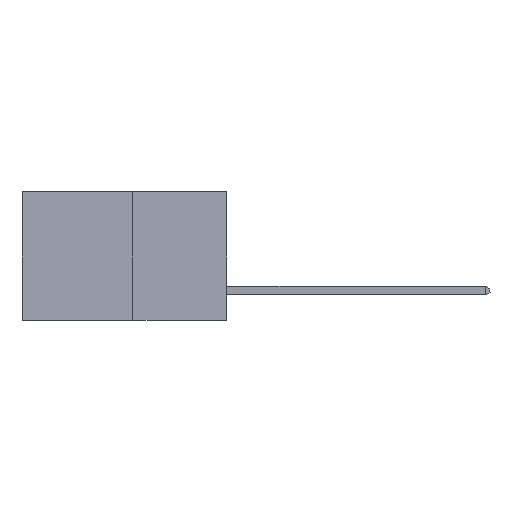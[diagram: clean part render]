
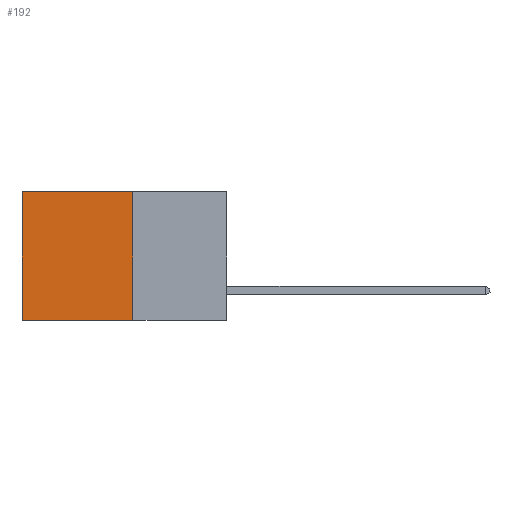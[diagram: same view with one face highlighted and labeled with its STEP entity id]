
A CAD part, left-side view. The second image highlights one B-rep face of the part: STEP entity #192.
In plain terms, the highlighted planar face has unit normal (-1, 0, 0).
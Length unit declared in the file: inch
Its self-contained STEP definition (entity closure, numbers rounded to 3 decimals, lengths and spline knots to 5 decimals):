
#144 = DIRECTION ( 'NONE',  ( 0., 0., -1. ) ) ;
#192 = ADVANCED_FACE ( 'NONE', ( #1609 ), #7700, .F. ) ;
#732 = EDGE_CURVE ( 'NONE', #3911, #3355, #3521, .T. ) ;
#922 = CARTESIAN_POINT ( 'NONE',  ( 0.277, 0.27, -0.37 ) ) ;
#1063 = CARTESIAN_POINT ( 'NONE',  ( 0.277, 0.59, -0.37 ) ) ;
#1507 = VERTEX_POINT ( 'NONE', #5740 ) ;
#1609 = FACE_OUTER_BOUND ( 'NONE', #6338, .T. ) ;
#2137 = LINE ( 'NONE', #7015, #6208 ) ;
#2222 = VECTOR ( 'NONE', #8670, 39.37008 ) ;
#3355 = VERTEX_POINT ( 'NONE', #5655 ) ;
#3521 = LINE ( 'NONE', #922, #7476 ) ;
#3780 = LINE ( 'NONE', #1063, #7697 ) ;
#3911 = VERTEX_POINT ( 'NONE', #6805 ) ;
#4600 = CARTESIAN_POINT ( 'NONE',  ( 0.277, 0.27, -0.37 ) ) ;
#5013 = ORIENTED_EDGE ( 'NONE', *, *, #8969, .T. ) ;
#5041 = CARTESIAN_POINT ( 'NONE',  ( 0.277, 0.27, 0. ) ) ;
#5655 = CARTESIAN_POINT ( 'NONE',  ( 0.277, 0.59, -0.37 ) ) ;
#5740 = CARTESIAN_POINT ( 'NONE',  ( 0.277, 0.27, 0. ) ) ;
#5811 = DIRECTION ( 'NONE',  ( 0., 0., -1. ) ) ;
#6208 = VECTOR ( 'NONE', #7864, 39.37008 ) ;
#6263 = AXIS2_PLACEMENT_3D ( 'NONE', #4600, #8094, #5811 ) ;
#6338 = EDGE_LOOP ( 'NONE', ( #5013, #8793, #6616, #9136 ) ) ;
#6616 = ORIENTED_EDGE ( 'NONE', *, *, #7579, .F. ) ;
#6711 = VERTEX_POINT ( 'NONE', #7146 ) ;
#6805 = CARTESIAN_POINT ( 'NONE',  ( 0.277, 0.27, -0.37 ) ) ;
#7010 = LINE ( 'NONE', #5041, #2222 ) ;
#7015 = CARTESIAN_POINT ( 'NONE',  ( 0.277, 0.27, -0.37 ) ) ;
#7146 = CARTESIAN_POINT ( 'NONE',  ( 0.277, 0.59, 0. ) ) ;
#7476 = VECTOR ( 'NONE', #8710, 39.37008 ) ;
#7579 = EDGE_CURVE ( 'NONE', #1507, #3911, #2137, .T. ) ;
#7697 = VECTOR ( 'NONE', #144, 39.37008 ) ;
#7700 = PLANE ( 'NONE',  #6263 ) ;
#7864 = DIRECTION ( 'NONE',  ( 0., 0., -1. ) ) ;
#8094 = DIRECTION ( 'NONE',  ( 1., 0., 0. ) ) ;
#8670 = DIRECTION ( 'NONE',  ( 0., 1., 0. ) ) ;
#8710 = DIRECTION ( 'NONE',  ( 0., 1., 0. ) ) ;
#8793 = ORIENTED_EDGE ( 'NONE', *, *, #732, .F. ) ;
#8969 = EDGE_CURVE ( 'NONE', #6711, #3355, #3780, .T. ) ;
#9136 = ORIENTED_EDGE ( 'NONE', *, *, #9675, .T. ) ;
#9675 = EDGE_CURVE ( 'NONE', #1507, #6711, #7010, .T. ) ;
